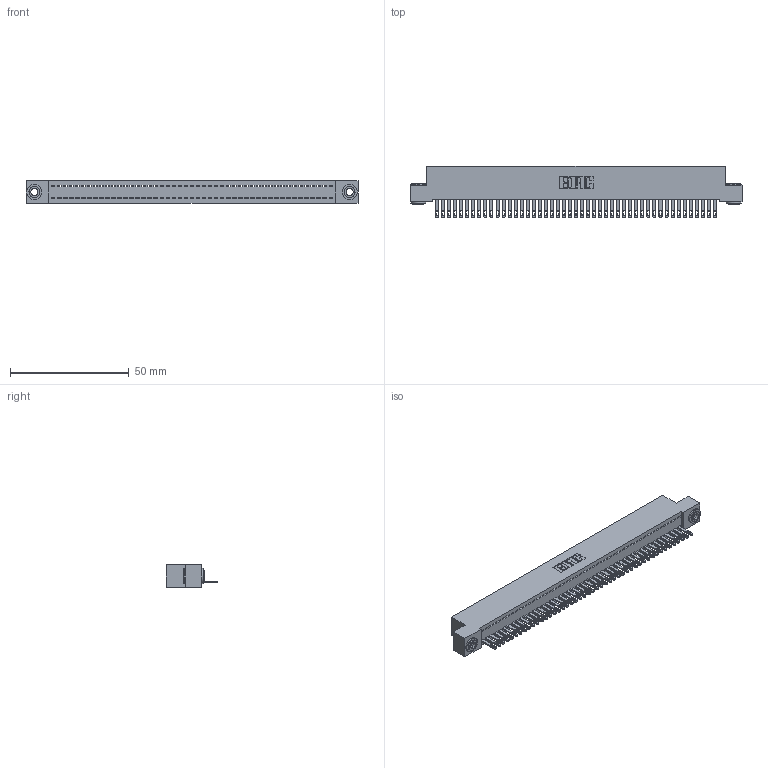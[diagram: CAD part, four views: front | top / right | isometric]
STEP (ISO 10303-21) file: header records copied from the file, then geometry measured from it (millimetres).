
FILE_DESCRIPTION (( 'STEP AP203' ), '1' );
FILE_NAME ('892-047-500-103.STEP', '2020-09-21T17:23:12', ( '' ), ( '' ), 'SwSTEP 2.0', 'SolidWorks 2020', '' );
FILE_SCHEMA (( 'CONFIG_CONTROL_DESIGN' ));
Length unit declared in the file: inch
Products named in the file (4): 342-250-002_345-250-002-102; 345-292-001_345-293-100; 892-047-500-103; 842 Part_.156 TH
Assembly tree (50 placements, depth 2):
  892-047-500-103
    842 Part_.156 TH
    345-292-001_345-293-100  x47
    342-250-002_345-250-002-102  x2
Bounding box: 139.7 x 21.85 x 9.4 mm (x, y, z)
Volume: 12319.2 mm3; surface area: 18502.3 mm2
Topology: 50 solids, 50 shells, 2686 faces, 8271 edges, 5510 vertices
Faces by surface type: plane 1768, cylinder 910, cone 8
Entity records: 28534 total; most frequent: CARTESIAN_POINT 4898, ORIENTED_EDGE 4874, DIRECTION 4157, EDGE_CURVE 2437, VECTOR 2281, LINE 2281, VERTEX_POINT 1622, AXIS2_PLACEMENT_3D 938
